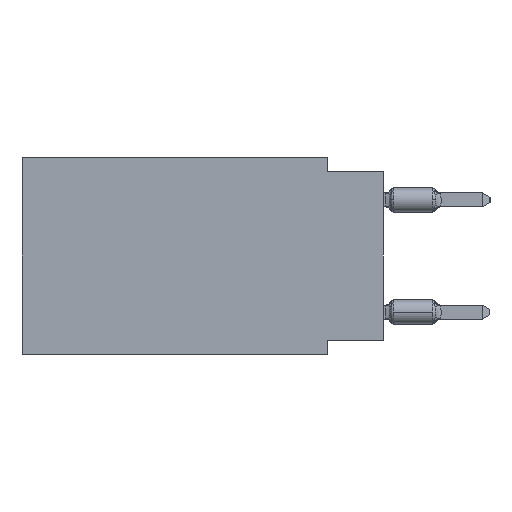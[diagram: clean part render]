
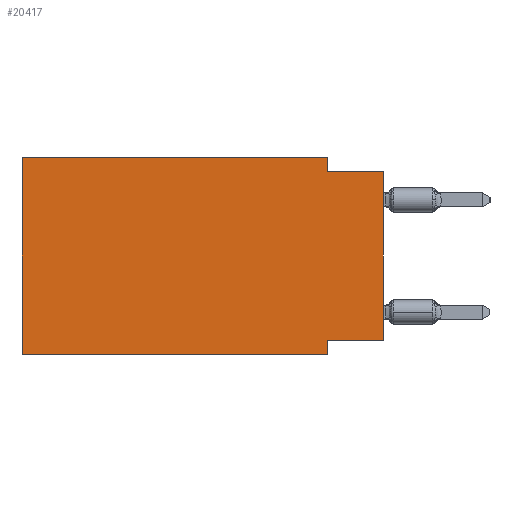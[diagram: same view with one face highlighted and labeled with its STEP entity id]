
A CAD part, left-side view. The second image highlights one B-rep face of the part: STEP entity #20417.
In plain terms, the highlighted planar face has unit normal (-1, 0, 0).
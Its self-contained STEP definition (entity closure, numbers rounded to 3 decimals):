
#486 = DIRECTION ( 'NONE',  ( 1., 0., 0. ) ) ;
#603 = EDGE_CURVE ( 'NONE', #10420, #32740, #33804, .T. ) ;
#1361 = CARTESIAN_POINT ( 'NONE',  ( 0., 2.54, 0. ) ) ;
#2431 = VECTOR ( 'NONE', #46426, 1000. ) ;
#2953 = DIRECTION ( 'NONE',  ( 0., 0., -1. ) ) ;
#3137 = EDGE_CURVE ( 'NONE', #7199, #10358, #17919, .T. ) ;
#5316 = LINE ( 'NONE', #20776, #48926 ) ;
#5790 = CARTESIAN_POINT ( 'NONE',  ( 0., 16.383, 0. ) ) ;
#7199 = VERTEX_POINT ( 'NONE', #34056 ) ;
#7939 = CARTESIAN_POINT ( 'NONE',  ( 0., 0., -0.635 ) ) ;
#9057 = ORIENTED_EDGE ( 'NONE', *, *, #28633, .F. ) ;
#9905 = EDGE_CURVE ( 'NONE', #37729, #7199, #29492, .T. ) ;
#10121 = VECTOR ( 'NONE', #29520, 1000. ) ;
#10358 = VERTEX_POINT ( 'NONE', #1361 ) ;
#10420 = VERTEX_POINT ( 'NONE', #22961 ) ;
#10431 = LINE ( 'NONE', #37989, #16424 ) ;
#11722 = LINE ( 'NONE', #31317, #30460 ) ;
#14994 = EDGE_CURVE ( 'NONE', #37729, #32740, #27391, .T. ) ;
#15870 = EDGE_CURVE ( 'NONE', #10358, #41278, #10431, .T. ) ;
#16097 = DIRECTION ( 'NONE',  ( 0., 0., 1. ) ) ;
#16353 = VECTOR ( 'NONE', #39501, 1000. ) ;
#16424 = VECTOR ( 'NONE', #2953, 1000. ) ;
#16447 = FACE_OUTER_BOUND ( 'NONE', #17596, .T. ) ;
#16699 = PLANE ( 'NONE',  #47631 ) ;
#17313 = ORIENTED_EDGE ( 'NONE', *, *, #3137, .F. ) ;
#17596 = EDGE_LOOP ( 'NONE', ( #24612, #9057, #48543, #17313, #19821, #34702, #32097, #32265 ) ) ;
#17919 = LINE ( 'NONE', #22802, #10121 ) ;
#18694 = VECTOR ( 'NONE', #21369, 1000. ) ;
#19821 = ORIENTED_EDGE ( 'NONE', *, *, #9905, .F. ) ;
#20417 = ADVANCED_FACE ( 'NONE', ( #16447 ), #16699, .F. ) ;
#20776 = CARTESIAN_POINT ( 'NONE',  ( 0., 0., -0.635 ) ) ;
#21369 = DIRECTION ( 'NONE',  ( 0., 1., 0. ) ) ;
#22200 = VERTEX_POINT ( 'NONE', #41403 ) ;
#22802 = CARTESIAN_POINT ( 'NONE',  ( 0., 16.383, 0. ) ) ;
#22961 = CARTESIAN_POINT ( 'NONE',  ( 0., 2.54, -8.255 ) ) ;
#24445 = CARTESIAN_POINT ( 'NONE',  ( 0., 2.54, -8.89 ) ) ;
#24612 = ORIENTED_EDGE ( 'NONE', *, *, #30085, .T. ) ;
#27391 = LINE ( 'NONE', #43109, #16353 ) ;
#28633 = EDGE_CURVE ( 'NONE', #41278, #36342, #5316, .T. ) ;
#28637 = VECTOR ( 'NONE', #49329, 1000. ) ;
#28823 = CARTESIAN_POINT ( 'NONE',  ( 0., 16.383, 0. ) ) ;
#29492 = LINE ( 'NONE', #5790, #28637 ) ;
#29520 = DIRECTION ( 'NONE',  ( 0., -1., 0. ) ) ;
#30085 = EDGE_CURVE ( 'NONE', #22200, #36342, #11722, .T. ) ;
#30460 = VECTOR ( 'NONE', #16097, 1000. ) ;
#30689 = CARTESIAN_POINT ( 'NONE',  ( 0., 2.54, -8.89 ) ) ;
#31317 = CARTESIAN_POINT ( 'NONE',  ( 0., 0., 0. ) ) ;
#32097 = ORIENTED_EDGE ( 'NONE', *, *, #603, .F. ) ;
#32118 = DIRECTION ( 'NONE',  ( 0., -1., 0. ) ) ;
#32265 = ORIENTED_EDGE ( 'NONE', *, *, #45448, .F. ) ;
#32673 = DIRECTION ( 'NONE',  ( 0., 0., -1. ) ) ;
#32740 = VERTEX_POINT ( 'NONE', #24445 ) ;
#33466 = LINE ( 'NONE', #48930, #18694 ) ;
#33804 = LINE ( 'NONE', #30689, #2431 ) ;
#34056 = CARTESIAN_POINT ( 'NONE',  ( 0., 16.383, 0. ) ) ;
#34702 = ORIENTED_EDGE ( 'NONE', *, *, #14994, .T. ) ;
#36342 = VERTEX_POINT ( 'NONE', #7939 ) ;
#37533 = CARTESIAN_POINT ( 'NONE',  ( 0., 2.54, -0.635 ) ) ;
#37729 = VERTEX_POINT ( 'NONE', #39736 ) ;
#37989 = CARTESIAN_POINT ( 'NONE',  ( 0., 2.54, 0. ) ) ;
#39501 = DIRECTION ( 'NONE',  ( 0., -1., 0. ) ) ;
#39736 = CARTESIAN_POINT ( 'NONE',  ( 0., 16.383, -8.89 ) ) ;
#41278 = VERTEX_POINT ( 'NONE', #37533 ) ;
#41403 = CARTESIAN_POINT ( 'NONE',  ( 0., 0., -8.255 ) ) ;
#43109 = CARTESIAN_POINT ( 'NONE',  ( 0., 16.383, -8.89 ) ) ;
#45448 = EDGE_CURVE ( 'NONE', #22200, #10420, #33466, .T. ) ;
#46426 = DIRECTION ( 'NONE',  ( 0., 0., -1. ) ) ;
#47631 = AXIS2_PLACEMENT_3D ( 'NONE', #28823, #486, #32673 ) ;
#48543 = ORIENTED_EDGE ( 'NONE', *, *, #15870, .F. ) ;
#48926 = VECTOR ( 'NONE', #32118, 1000. ) ;
#48930 = CARTESIAN_POINT ( 'NONE',  ( 0., 0., -8.255 ) ) ;
#49329 = DIRECTION ( 'NONE',  ( 0., 0., 1. ) ) ;
